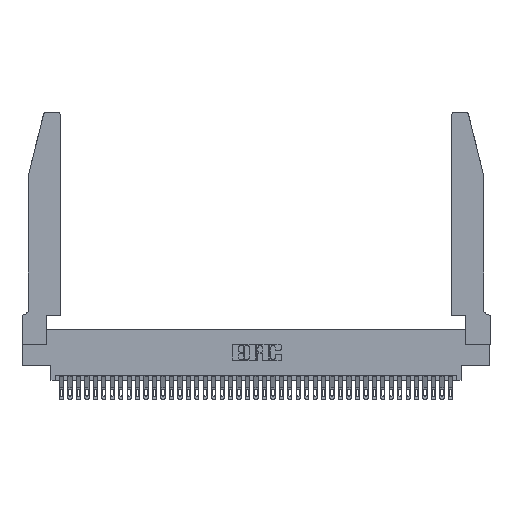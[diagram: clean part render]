
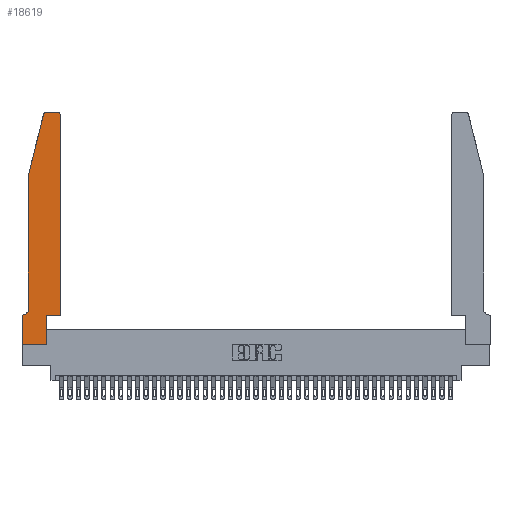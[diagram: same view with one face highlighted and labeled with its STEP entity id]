
A CAD part, top view. The second image highlights one B-rep face of the part: STEP entity #18619.
In plain terms, the highlighted planar face has unit normal (0, 0, 1).
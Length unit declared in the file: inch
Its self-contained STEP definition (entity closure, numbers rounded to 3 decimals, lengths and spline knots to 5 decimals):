
#376 = CARTESIAN_POINT ( 'NONE',  ( 0.4505, 0.35, 0.37 ) ) ;
#763 = AXIS2_PLACEMENT_3D ( 'NONE', #16674, #38840, #19913 ) ;
#1151 = DIRECTION ( 'NONE',  ( 1., 0., 0. ) ) ;
#1626 = ORIENTED_EDGE ( 'NONE', *, *, #10692, .T. ) ;
#3017 = CARTESIAN_POINT ( 'NONE',  ( 0.284, 2.72, 0.37 ) ) ;
#3197 = DIRECTION ( 'NONE',  ( -1., 0., 0. ) ) ;
#3318 = CARTESIAN_POINT ( 'NONE',  ( 0.4505, 0.35, 0.37 ) ) ;
#4191 = CARTESIAN_POINT ( 'NONE',  ( 0.0755, 2., 0.37 ) ) ;
#4648 = CARTESIAN_POINT ( 'NONE',  ( 0.25487, 2.72718, 0.37 ) ) ;
#4739 = EDGE_LOOP ( 'NONE', ( #37549, #17270, #34078, #11780, #37039, #38084, #22284, #1626, #18819, #35592, #14277, #39604 ) ) ;
#4901 = VECTOR ( 'NONE', #37767, 39.37008 ) ;
#5777 = CIRCLE ( 'NONE', #763, 0.03 ) ;
#6294 = DIRECTION ( 'NONE',  ( 1., 0., 0. ) ) ;
#8982 = CARTESIAN_POINT ( 'NONE',  ( 0.0055, 0.42, 0.37 ) ) ;
#9508 = VECTOR ( 'NONE', #28894, 39.37008 ) ;
#10394 = VERTEX_POINT ( 'NONE', #41263 ) ;
#10692 = EDGE_CURVE ( 'NONE', #25076, #24492, #21491, .T. ) ;
#10921 = EDGE_CURVE ( 'NONE', #10394, #41187, #13499, .T. ) ;
#10946 = AXIS2_PLACEMENT_3D ( 'NONE', #8982, #31205, #12231 ) ;
#10969 = FACE_OUTER_BOUND ( 'NONE', #4739, .T. ) ;
#11780 = ORIENTED_EDGE ( 'NONE', *, *, #27026, .T. ) ;
#12231 = DIRECTION ( 'NONE',  ( -1., 0., 0. ) ) ;
#12877 = CARTESIAN_POINT ( 'NONE',  ( 0.2605, 2.75, 0.37 ) ) ;
#12908 = DIRECTION ( 'NONE',  ( 0., -1., 0. ) ) ;
#13439 = VECTOR ( 'NONE', #22602, 39.37008 ) ;
#13499 = CIRCLE ( 'NONE', #10946, 0.07 ) ;
#13716 = VECTOR ( 'NONE', #26562, 39.37008 ) ;
#14168 = CARTESIAN_POINT ( 'NONE',  ( 0., 0., 0.37 ) ) ;
#14277 = ORIENTED_EDGE ( 'NONE', *, *, #21941, .T. ) ;
#14494 = LINE ( 'NONE', #25197, #4901 ) ;
#15394 = LINE ( 'NONE', #3318, #13439 ) ;
#15874 = VERTEX_POINT ( 'NONE', #28045 ) ;
#16194 = VERTEX_POINT ( 'NONE', #36304 ) ;
#16674 = CARTESIAN_POINT ( 'NONE',  ( 0.4205, 2.72, 0.37 ) ) ;
#16850 = VERTEX_POINT ( 'NONE', #39363 ) ;
#16910 = VERTEX_POINT ( 'NONE', #4648 ) ;
#17114 = EDGE_CURVE ( 'NONE', #41187, #20991, #31941, .T. ) ;
#17270 = ORIENTED_EDGE ( 'NONE', *, *, #29288, .T. ) ;
#18291 = LINE ( 'NONE', #33491, #34085 ) ;
#18619 = ADVANCED_FACE ( 'NONE', ( #10969 ), #38109, .T. ) ;
#18819 = ORIENTED_EDGE ( 'NONE', *, *, #33367, .T. ) ;
#19179 = AXIS2_PLACEMENT_3D ( 'NONE', #37969, #41317, #22374 ) ;
#19280 = EDGE_CURVE ( 'NONE', #16194, #36076, #15394, .T. ) ;
#19848 = VECTOR ( 'NONE', #12908, 39.37008 ) ;
#19913 = DIRECTION ( 'NONE',  ( 1., 0., 0. ) ) ;
#20180 = VERTEX_POINT ( 'NONE', #27175 ) ;
#20587 = LINE ( 'NONE', #12877, #26959 ) ;
#20971 = DIRECTION ( 'NONE',  ( 0., 1., 0. ) ) ;
#20991 = VERTEX_POINT ( 'NONE', #24756 ) ;
#21213 = LINE ( 'NONE', #4191, #13716 ) ;
#21491 = LINE ( 'NONE', #14168, #30844 ) ;
#21679 = EDGE_CURVE ( 'NONE', #20991, #25076, #37600, .T. ) ;
#21941 = EDGE_CURVE ( 'NONE', #36076, #20180, #18291, .T. ) ;
#22284 = ORIENTED_EDGE ( 'NONE', *, *, #21679, .T. ) ;
#22374 = DIRECTION ( 'NONE',  ( 1., 0., 0. ) ) ;
#22602 = DIRECTION ( 'NONE',  ( 1., 0., 0. ) ) ;
#23554 = VECTOR ( 'NONE', #40721, 39.37008 ) ;
#24492 = VERTEX_POINT ( 'NONE', #41338 ) ;
#24756 = CARTESIAN_POINT ( 'NONE',  ( 0., 0.35, 0.37 ) ) ;
#25076 = VERTEX_POINT ( 'NONE', #37944 ) ;
#25197 = CARTESIAN_POINT ( 'NONE',  ( 0.0755, 2., 0.37 ) ) ;
#25332 = VERTEX_POINT ( 'NONE', #36504 ) ;
#25437 = DIRECTION ( 'NONE',  ( 0., 0., 1. ) ) ;
#25588 = EDGE_CURVE ( 'NONE', #16910, #15874, #14494, .T. ) ;
#25817 = CARTESIAN_POINT ( 'NONE',  ( 0.0055, 0.35, 0.37 ) ) ;
#26413 = LINE ( 'NONE', #38465, #9508 ) ;
#26562 = DIRECTION ( 'NONE',  ( 0., -1., 0. ) ) ;
#26959 = VECTOR ( 'NONE', #3197, 39.37008 ) ;
#27026 = EDGE_CURVE ( 'NONE', #15874, #10394, #21213, .T. ) ;
#27175 = CARTESIAN_POINT ( 'NONE',  ( 0.4505, 2.72, 0.37 ) ) ;
#28045 = CARTESIAN_POINT ( 'NONE',  ( 0.0755, 2., 0.37 ) ) ;
#28650 = AXIS2_PLACEMENT_3D ( 'NONE', #3017, #25437, #6294 ) ;
#28894 = DIRECTION ( 'NONE',  ( 0., 1., 0. ) ) ;
#29288 = EDGE_CURVE ( 'NONE', #16850, #16910, #40368, .T. ) ;
#30844 = VECTOR ( 'NONE', #1151, 39.37008 ) ;
#31205 = DIRECTION ( 'NONE',  ( 0., 0., -1. ) ) ;
#31809 = EDGE_CURVE ( 'NONE', #20180, #25332, #5777, .T. ) ;
#31941 = LINE ( 'NONE', #37504, #23554 ) ;
#32655 = EDGE_CURVE ( 'NONE', #25332, #16850, #20587, .T. ) ;
#33367 = EDGE_CURVE ( 'NONE', #24492, #16194, #26413, .T. ) ;
#33491 = CARTESIAN_POINT ( 'NONE',  ( 0.4505, 0.35, 0.37 ) ) ;
#34078 = ORIENTED_EDGE ( 'NONE', *, *, #25588, .T. ) ;
#34085 = VECTOR ( 'NONE', #20971, 39.37008 ) ;
#35039 = CARTESIAN_POINT ( 'NONE',  ( 0., 0., 0.37 ) ) ;
#35592 = ORIENTED_EDGE ( 'NONE', *, *, #19280, .T. ) ;
#36076 = VERTEX_POINT ( 'NONE', #376 ) ;
#36304 = CARTESIAN_POINT ( 'NONE',  ( 0.2865, 0.35, 0.37 ) ) ;
#36504 = CARTESIAN_POINT ( 'NONE',  ( 0.4205, 2.75, 0.37 ) ) ;
#37039 = ORIENTED_EDGE ( 'NONE', *, *, #10921, .T. ) ;
#37504 = CARTESIAN_POINT ( 'NONE',  ( 0.0755, 0.35, 0.37 ) ) ;
#37549 = ORIENTED_EDGE ( 'NONE', *, *, #32655, .T. ) ;
#37600 = LINE ( 'NONE', #35039, #19848 ) ;
#37767 = DIRECTION ( 'NONE',  ( -0.239, -0.971, 0. ) ) ;
#37944 = CARTESIAN_POINT ( 'NONE',  ( 0., 0., 0.37 ) ) ;
#37969 = CARTESIAN_POINT ( 'NONE',  ( 0., 0.35, 0.37 ) ) ;
#38084 = ORIENTED_EDGE ( 'NONE', *, *, #17114, .T. ) ;
#38109 = PLANE ( 'NONE',  #19179 ) ;
#38465 = CARTESIAN_POINT ( 'NONE',  ( 0.2865, 0.35, 0.37 ) ) ;
#38840 = DIRECTION ( 'NONE',  ( 0., 0., 1. ) ) ;
#39363 = CARTESIAN_POINT ( 'NONE',  ( 0.284, 2.75, 0.37 ) ) ;
#39604 = ORIENTED_EDGE ( 'NONE', *, *, #31809, .T. ) ;
#40368 = CIRCLE ( 'NONE', #28650, 0.03 ) ;
#40721 = DIRECTION ( 'NONE',  ( -1., 0., 0. ) ) ;
#41187 = VERTEX_POINT ( 'NONE', #25817 ) ;
#41263 = CARTESIAN_POINT ( 'NONE',  ( 0.0755, 0.42, 0.37 ) ) ;
#41317 = DIRECTION ( 'NONE',  ( 0., 0., 1. ) ) ;
#41338 = CARTESIAN_POINT ( 'NONE',  ( 0.2865, 0., 0.37 ) ) ;
